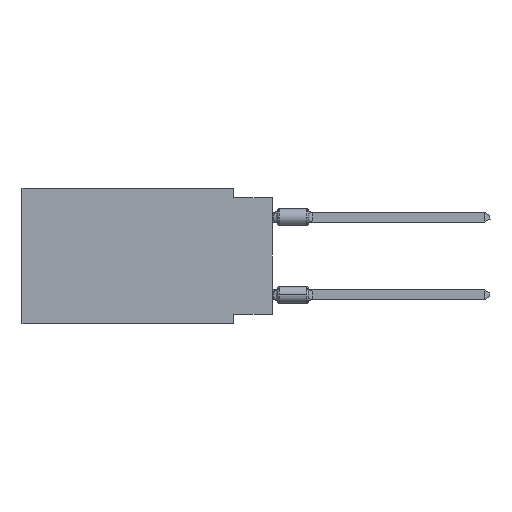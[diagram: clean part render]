
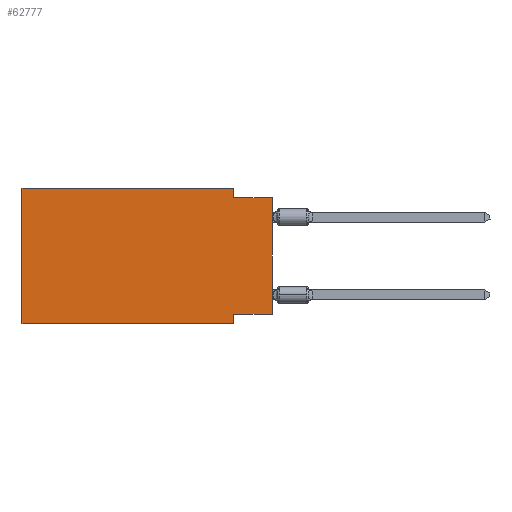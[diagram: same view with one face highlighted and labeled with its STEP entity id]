
A CAD part, left-side view. The second image highlights one B-rep face of the part: STEP entity #62777.
In plain terms, the highlighted planar face has unit normal (-1, 0, 0).
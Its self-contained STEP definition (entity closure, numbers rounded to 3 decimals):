
#2035 = PLANE ( 'NONE',  #73075 ) ;
#2787 = EDGE_LOOP ( 'NONE', ( #8548, #47899, #13513, #6973, #30108, #3166, #38626, #66397 ) ) ;
#3166 = ORIENTED_EDGE ( 'NONE', *, *, #16663, .T. ) ;
#6205 = VERTEX_POINT ( 'NONE', #12382 ) ;
#6973 = ORIENTED_EDGE ( 'NONE', *, *, #68606, .F. ) ;
#8165 = VECTOR ( 'NONE', #31092, 1000. ) ;
#8548 = ORIENTED_EDGE ( 'NONE', *, *, #18116, .T. ) ;
#10915 = VERTEX_POINT ( 'NONE', #24731 ) ;
#12382 = CARTESIAN_POINT ( 'NONE',  ( 0., 16.383, -8.89 ) ) ;
#12472 = CARTESIAN_POINT ( 'NONE',  ( 0., 0., -0.635 ) ) ;
#13212 = FACE_OUTER_BOUND ( 'NONE', #2787, .T. ) ;
#13513 = ORIENTED_EDGE ( 'NONE', *, *, #42265, .F. ) ;
#14193 = LINE ( 'NONE', #70791, #66114 ) ;
#16663 = EDGE_CURVE ( 'NONE', #6205, #10915, #51412, .T. ) ;
#18116 = EDGE_CURVE ( 'NONE', #32197, #47362, #14193, .T. ) ;
#18158 = VERTEX_POINT ( 'NONE', #64862 ) ;
#20671 = EDGE_CURVE ( 'NONE', #6205, #55080, #70786, .T. ) ;
#24182 = CARTESIAN_POINT ( 'NONE',  ( 0., 16.383, -8.89 ) ) ;
#24731 = CARTESIAN_POINT ( 'NONE',  ( 0., 2.54, -8.89 ) ) ;
#24752 = CARTESIAN_POINT ( 'NONE',  ( 0., 16.383, 0. ) ) ;
#26910 = CARTESIAN_POINT ( 'NONE',  ( 0., 16.383, 0. ) ) ;
#30108 = ORIENTED_EDGE ( 'NONE', *, *, #20671, .F. ) ;
#31092 = DIRECTION ( 'NONE',  ( 0., 0., -1. ) ) ;
#31352 = VECTOR ( 'NONE', #66067, 1000. ) ;
#31829 = LINE ( 'NONE', #71638, #31352 ) ;
#32197 = VERTEX_POINT ( 'NONE', #40282 ) ;
#32402 = CARTESIAN_POINT ( 'NONE',  ( 0., 16.383, 0. ) ) ;
#33352 = LINE ( 'NONE', #66851, #67440 ) ;
#34790 = EDGE_CURVE ( 'NONE', #32197, #18158, #55100, .T. ) ;
#36500 = CARTESIAN_POINT ( 'NONE',  ( 0., 2.54, -8.89 ) ) ;
#38626 = ORIENTED_EDGE ( 'NONE', *, *, #63657, .F. ) ;
#39921 = VECTOR ( 'NONE', #48752, 1000. ) ;
#40282 = CARTESIAN_POINT ( 'NONE',  ( 0., 0., -8.255 ) ) ;
#40527 = LINE ( 'NONE', #60118, #8165 ) ;
#42265 = EDGE_CURVE ( 'NONE', #68293, #56666, #40527, .T. ) ;
#43170 = LINE ( 'NONE', #36500, #39921 ) ;
#43227 = DIRECTION ( 'NONE',  ( 0., 0., 1. ) ) ;
#47362 = VERTEX_POINT ( 'NONE', #12472 ) ;
#47899 = ORIENTED_EDGE ( 'NONE', *, *, #65307, .F. ) ;
#48167 = VECTOR ( 'NONE', #52155, 1000. ) ;
#48752 = DIRECTION ( 'NONE',  ( 0., 0., -1. ) ) ;
#49512 = CARTESIAN_POINT ( 'NONE',  ( 0., 0., -8.255 ) ) ;
#49755 = VECTOR ( 'NONE', #72220, 1000. ) ;
#50475 = DIRECTION ( 'NONE',  ( 0., -1., 0. ) ) ;
#51121 = CARTESIAN_POINT ( 'NONE',  ( 0., 2.54, -0.635 ) ) ;
#51412 = LINE ( 'NONE', #24182, #48167 ) ;
#52155 = DIRECTION ( 'NONE',  ( 0., -1., 0. ) ) ;
#53802 = DIRECTION ( 'NONE',  ( 1., 0., 0. ) ) ;
#55080 = VERTEX_POINT ( 'NONE', #26910 ) ;
#55100 = LINE ( 'NONE', #49512, #49755 ) ;
#56666 = VERTEX_POINT ( 'NONE', #51121 ) ;
#59123 = VECTOR ( 'NONE', #43227, 1000. ) ;
#60118 = CARTESIAN_POINT ( 'NONE',  ( 0., 2.54, 0. ) ) ;
#60935 = CARTESIAN_POINT ( 'NONE',  ( 0., 2.54, 0. ) ) ;
#62777 = ADVANCED_FACE ( 'NONE', ( #13212 ), #2035, .F. ) ;
#63657 = EDGE_CURVE ( 'NONE', #18158, #10915, #43170, .T. ) ;
#64862 = CARTESIAN_POINT ( 'NONE',  ( 0., 2.54, -8.255 ) ) ;
#65307 = EDGE_CURVE ( 'NONE', #56666, #47362, #33352, .T. ) ;
#66067 = DIRECTION ( 'NONE',  ( 0., -1., 0. ) ) ;
#66114 = VECTOR ( 'NONE', #71871, 1000. ) ;
#66397 = ORIENTED_EDGE ( 'NONE', *, *, #34790, .F. ) ;
#66851 = CARTESIAN_POINT ( 'NONE',  ( 0., 0., -0.635 ) ) ;
#67440 = VECTOR ( 'NONE', #50475, 1000. ) ;
#68293 = VERTEX_POINT ( 'NONE', #60935 ) ;
#68606 = EDGE_CURVE ( 'NONE', #55080, #68293, #31829, .T. ) ;
#70786 = LINE ( 'NONE', #32402, #59123 ) ;
#70791 = CARTESIAN_POINT ( 'NONE',  ( 0., 0., 0. ) ) ;
#71621 = DIRECTION ( 'NONE',  ( 0., 0., -1. ) ) ;
#71638 = CARTESIAN_POINT ( 'NONE',  ( 0., 16.383, 0. ) ) ;
#71871 = DIRECTION ( 'NONE',  ( 0., 0., 1. ) ) ;
#72220 = DIRECTION ( 'NONE',  ( 0., 1., 0. ) ) ;
#73075 = AXIS2_PLACEMENT_3D ( 'NONE', #24752, #53802, #71621 ) ;
